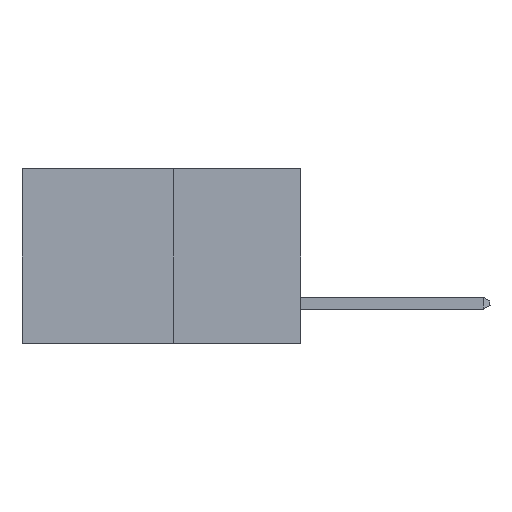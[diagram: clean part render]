
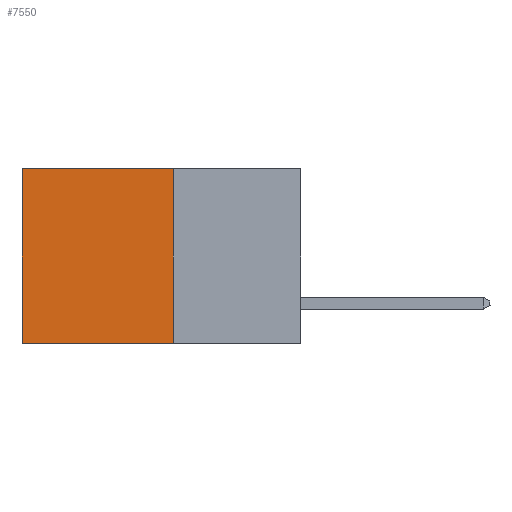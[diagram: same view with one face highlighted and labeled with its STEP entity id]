
A CAD part, left-side view. The second image highlights one B-rep face of the part: STEP entity #7550.
In plain terms, the highlighted planar face has unit normal (-1, 0, 0).
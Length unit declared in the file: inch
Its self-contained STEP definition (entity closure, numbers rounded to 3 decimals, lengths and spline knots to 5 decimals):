
#1835 = VECTOR ( 'NONE', #11639, 39.37008 ) ;
#1941 = DIRECTION ( 'NONE',  ( 0., 0., -1. ) ) ;
#1995 = CARTESIAN_POINT ( 'NONE',  ( 0.277, 0.27, -0.37 ) ) ;
#2093 = EDGE_CURVE ( 'NONE', #7816, #17953, #4815, .T. ) ;
#2602 = ORIENTED_EDGE ( 'NONE', *, *, #12457, .F. ) ;
#2728 = LINE ( 'NONE', #6242, #19059 ) ;
#4502 = CARTESIAN_POINT ( 'NONE',  ( 0.277, 0.59, 0. ) ) ;
#4815 = LINE ( 'NONE', #18585, #8631 ) ;
#5297 = DIRECTION ( 'NONE',  ( 1., 0., 0. ) ) ;
#6141 = LINE ( 'NONE', #8392, #9946 ) ;
#6242 = CARTESIAN_POINT ( 'NONE',  ( 0.277, 0.59, -0.37 ) ) ;
#7550 = ADVANCED_FACE ( 'NONE', ( #14305 ), #14839, .F. ) ;
#7816 = VERTEX_POINT ( 'NONE', #13892 ) ;
#8200 = CARTESIAN_POINT ( 'NONE',  ( 0.277, 0.59, -0.37 ) ) ;
#8392 = CARTESIAN_POINT ( 'NONE',  ( 0.277, 0.27, -0.37 ) ) ;
#8631 = VECTOR ( 'NONE', #10882, 39.37008 ) ;
#8883 = ORIENTED_EDGE ( 'NONE', *, *, #9209, .T. ) ;
#9209 = EDGE_CURVE ( 'NONE', #17953, #11170, #2728, .T. ) ;
#9946 = VECTOR ( 'NONE', #1941, 39.37008 ) ;
#10577 = ORIENTED_EDGE ( 'NONE', *, *, #2093, .T. ) ;
#10882 = DIRECTION ( 'NONE',  ( 0., 1., 0. ) ) ;
#11170 = VERTEX_POINT ( 'NONE', #8200 ) ;
#11639 = DIRECTION ( 'NONE',  ( 0., 1., 0. ) ) ;
#11697 = CARTESIAN_POINT ( 'NONE',  ( 0.277, 0.27, -0.37 ) ) ;
#12457 = EDGE_CURVE ( 'NONE', #16187, #11170, #18196, .T. ) ;
#12684 = DIRECTION ( 'NONE',  ( 0., 0., -1. ) ) ;
#13892 = CARTESIAN_POINT ( 'NONE',  ( 0.277, 0.27, 0. ) ) ;
#14305 = FACE_OUTER_BOUND ( 'NONE', #16549, .T. ) ;
#14366 = CARTESIAN_POINT ( 'NONE',  ( 0.277, 0.27, -0.37 ) ) ;
#14839 = PLANE ( 'NONE',  #18618 ) ;
#16187 = VERTEX_POINT ( 'NONE', #14366 ) ;
#16387 = DIRECTION ( 'NONE',  ( 0., 0., -1. ) ) ;
#16549 = EDGE_LOOP ( 'NONE', ( #8883, #2602, #17827, #10577 ) ) ;
#16984 = EDGE_CURVE ( 'NONE', #7816, #16187, #6141, .T. ) ;
#17827 = ORIENTED_EDGE ( 'NONE', *, *, #16984, .F. ) ;
#17953 = VERTEX_POINT ( 'NONE', #4502 ) ;
#18196 = LINE ( 'NONE', #1995, #1835 ) ;
#18585 = CARTESIAN_POINT ( 'NONE',  ( 0.277, 0.27, 0. ) ) ;
#18618 = AXIS2_PLACEMENT_3D ( 'NONE', #11697, #5297, #16387 ) ;
#19059 = VECTOR ( 'NONE', #12684, 39.37008 ) ;
